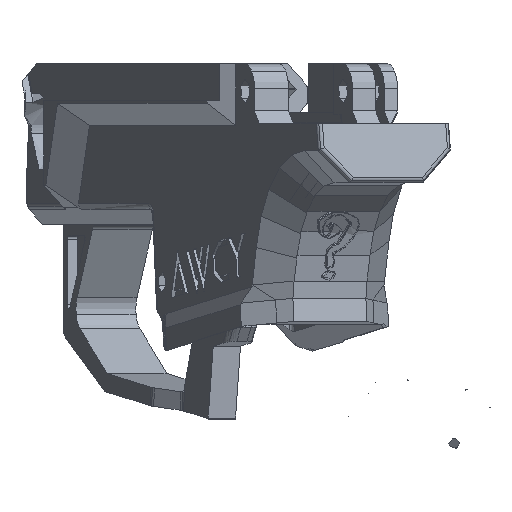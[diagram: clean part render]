
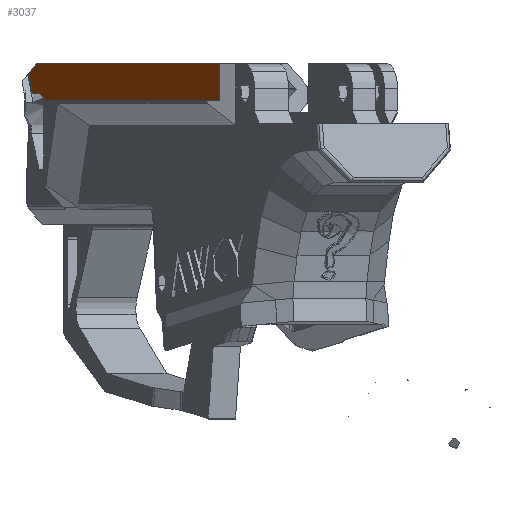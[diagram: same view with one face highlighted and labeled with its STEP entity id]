
A CAD part, front view. The second image highlights one B-rep face of the part: STEP entity #3037.
In plain terms, the highlighted face is planar.
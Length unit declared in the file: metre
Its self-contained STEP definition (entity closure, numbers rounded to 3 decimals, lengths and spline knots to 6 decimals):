
#3037=ADVANCED_FACE('0:1592',(#6528),#6529,.T.);
#6528=FACE_OUTER_BOUND('',#11681,.T.);
#6529=PLANE('',#11682);
#11681=EDGE_LOOP('',(#24725,#24726,#24727,#24728,#24729,#24730,#24731,#24732));
#11682=AXIS2_PLACEMENT_3D('',#24733,#24734,#24735);
#24725=ORIENTED_EDGE('',*,*,#33476,.T.);
#24726=ORIENTED_EDGE('',*,*,#30628,.F.);
#24727=ORIENTED_EDGE('',*,*,#33485,.T.);
#24728=ORIENTED_EDGE('',*,*,#33486,.T.);
#24729=ORIENTED_EDGE('',*,*,#33487,.T.);
#24730=ORIENTED_EDGE('',*,*,#33488,.T.);
#24731=ORIENTED_EDGE('',*,*,#33439,.T.);
#24732=ORIENTED_EDGE('',*,*,#33483,.T.);
#24733=CARTESIAN_POINT('',(-0.003858,-0.03552,0.072791));
#24734=DIRECTION('',(0.,-1.0,0.));
#24735=DIRECTION('',(0.0,0.,-1.0));
#30628=EDGE_CURVE('0:2329',#35752,#35754,#35755,.T.);
#33439=EDGE_CURVE('0:7195',#40469,#40467,#40470,.T.);
#33476=EDGE_CURVE('0:7306',#40522,#35754,#40524,.T.);
#33483=EDGE_CURVE('0:7327',#40467,#40522,#40534,.T.);
#33485=EDGE_CURVE('0:7333',#35752,#40536,#40537,.T.);
#33486=EDGE_CURVE('0:7336',#40536,#40538,#40539,.T.);
#33487=EDGE_CURVE('0:7339',#40538,#40540,#40541,.T.);
#33488=EDGE_CURVE('0:7342',#40540,#40469,#40542,.T.);
#35752=VERTEX_POINT('',#43790);
#35754=VERTEX_POINT('',#43792);
#35755=CIRCLE('',#43793,0.008847);
#40467=VERTEX_POINT('',#52013);
#40469=VERTEX_POINT('',#52016);
#40470=LINE('',#52017,#52018);
#40522=VERTEX_POINT('',#52115);
#40524=LINE('',#52118,#52119);
#40534=LINE('',#52151,#52152);
#40536=VERTEX_POINT('',#52155);
#40537=LINE('',#52156,#52157);
#40538=VERTEX_POINT('',#52158);
#40539=LINE('',#52159,#52160);
#40540=VERTEX_POINT('',#52161);
#40541=LINE('',#52162,#52163);
#40542=LINE('',#52164,#52165);
#43790=CARTESIAN_POINT('',(-0.052092,-0.03552,0.066051));
#43792=CARTESIAN_POINT('',(-0.061985,-0.03552,0.070216));
#43793=AXIS2_PLACEMENT_3D('',#58871,#58872,#58873);
#52013=CARTESIAN_POINT('',(-0.059398,-0.03552,0.076683));
#52016=CARTESIAN_POINT('',(0.041375,-0.03552,0.076683));
#52017=CARTESIAN_POINT('',(0.020902,-0.03552,0.076683));
#52018=VECTOR('',#62784,0.01);
#52115=CARTESIAN_POINT('',(-0.063996,-0.03552,0.074532));
#52118=CARTESIAN_POINT('',(-0.058661,-0.03552,0.063084));
#52119=VECTOR('',#62819,0.01);
#52151=CARTESIAN_POINT('',(-0.069333,-0.03552,0.072036));
#52152=VECTOR('',#62824,0.01);
#52155=CARTESIAN_POINT('',(-0.050814,-0.03552,0.066051));
#52156=CARTESIAN_POINT('',(-0.036074,-0.03552,0.066051));
#52157=VECTOR('',#62826,0.01);
#52158=CARTESIAN_POINT('',(-0.050814,-0.03552,0.068686));
#52159=CARTESIAN_POINT('',(-0.050814,-0.03552,0.059317));
#52160=VECTOR('',#62827,0.01);
#52161=CARTESIAN_POINT('',(0.041375,-0.03552,0.068686));
#52162=CARTESIAN_POINT('',(-0.003748,-0.03552,0.068686));
#52163=VECTOR('',#62828,0.01);
#52164=CARTESIAN_POINT('',(0.041375,-0.03552,0.068686));
#52165=VECTOR('',#62829,0.01);
#58871=CARTESIAN_POINT('',(-0.059768,-0.03552,0.061651));
#58872=DIRECTION('',(0.,-1.0,0.));
#58873=DIRECTION('',(1.0,0.,0.));
#62784=DIRECTION('',(-1.0,0.,0.));
#62819=DIRECTION('',(0.422,0.,-0.906));
#62824=DIRECTION('',(-0.906,0.,-0.424));
#62826=DIRECTION('',(1.,0.,0.));
#62827=DIRECTION('',(0.,0.,1.0));
#62828=DIRECTION('',(1.0,0.,0.));
#62829=DIRECTION('',(0.,0.,1.0));
